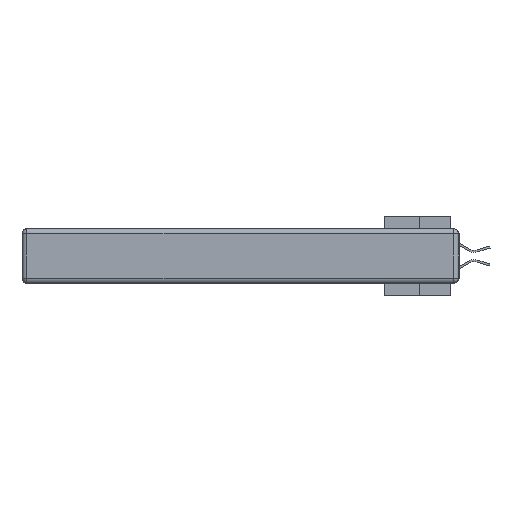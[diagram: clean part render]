
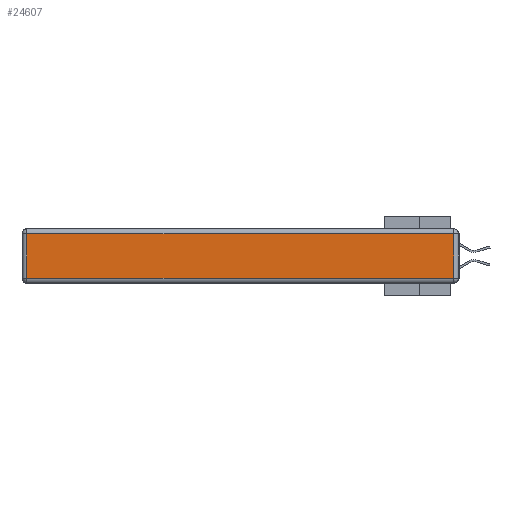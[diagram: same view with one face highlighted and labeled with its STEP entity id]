
A CAD part, left-side view. The second image highlights one B-rep face of the part: STEP entity #24607.
In plain terms, the highlighted planar face has unit normal (-1, 0, 0).
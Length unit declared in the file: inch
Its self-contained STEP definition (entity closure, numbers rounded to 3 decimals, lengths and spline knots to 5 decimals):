
#2348 = ORIENTED_EDGE ( 'NONE', *, *, #29073, .T. ) ;
#2840 = CARTESIAN_POINT ( 'NONE',  ( 0., 2.72, -0.343 ) ) ;
#3123 = CARTESIAN_POINT ( 'NONE',  ( 0., 2.72, -0.313 ) ) ;
#3370 = CARTESIAN_POINT ( 'NONE',  ( 0., 0., -0.343 ) ) ;
#4857 = LINE ( 'NONE', #33003, #16143 ) ;
#6246 = CARTESIAN_POINT ( 'NONE',  ( 0., 2.72, -0.03 ) ) ;
#7114 = VERTEX_POINT ( 'NONE', #3123 ) ;
#9445 = DIRECTION ( 'NONE',  ( 0., 1., 0. ) ) ;
#12820 = VECTOR ( 'NONE', #31341, 39.37008 ) ;
#13933 = EDGE_CURVE ( 'NONE', #24529, #7114, #23409, .T. ) ;
#14555 = EDGE_CURVE ( 'NONE', #23096, #25007, #15583, .T. ) ;
#15583 = LINE ( 'NONE', #30411, #22981 ) ;
#16143 = VECTOR ( 'NONE', #22887, 39.37008 ) ;
#16376 = ORIENTED_EDGE ( 'NONE', *, *, #13933, .T. ) ;
#17483 = CARTESIAN_POINT ( 'NONE',  ( 0., 0.03, -0.313 ) ) ;
#19044 = EDGE_CURVE ( 'NONE', #25007, #24529, #22059, .T. ) ;
#20258 = EDGE_LOOP ( 'NONE', ( #2348, #28731, #32077, #16376 ) ) ;
#20476 = CARTESIAN_POINT ( 'NONE',  ( 0., 2.75, -0.03 ) ) ;
#21233 = FACE_OUTER_BOUND ( 'NONE', #20258, .T. ) ;
#21402 = DIRECTION ( 'NONE',  ( -1., 0., 0. ) ) ;
#22059 = LINE ( 'NONE', #20476, #31390 ) ;
#22887 = DIRECTION ( 'NONE',  ( 0., -1., 0. ) ) ;
#22981 = VECTOR ( 'NONE', #25879, 39.37008 ) ;
#23096 = VERTEX_POINT ( 'NONE', #17483 ) ;
#23409 = LINE ( 'NONE', #2840, #12820 ) ;
#24529 = VERTEX_POINT ( 'NONE', #6246 ) ;
#24607 = ADVANCED_FACE ( 'NONE', ( #21233 ), #26481, .T. ) ;
#24687 = CARTESIAN_POINT ( 'NONE',  ( 0., 0.03, -0.03 ) ) ;
#25007 = VERTEX_POINT ( 'NONE', #24687 ) ;
#25879 = DIRECTION ( 'NONE',  ( 0., 0., 1. ) ) ;
#26481 = PLANE ( 'NONE',  #31069 ) ;
#28731 = ORIENTED_EDGE ( 'NONE', *, *, #14555, .T. ) ;
#29073 = EDGE_CURVE ( 'NONE', #7114, #23096, #4857, .T. ) ;
#29979 = DIRECTION ( 'NONE',  ( 0., 0., 1. ) ) ;
#30411 = CARTESIAN_POINT ( 'NONE',  ( 0., 0.03, -0.343 ) ) ;
#31069 = AXIS2_PLACEMENT_3D ( 'NONE', #3370, #21402, #29979 ) ;
#31341 = DIRECTION ( 'NONE',  ( 0., 0., -1. ) ) ;
#31390 = VECTOR ( 'NONE', #9445, 39.37008 ) ;
#32077 = ORIENTED_EDGE ( 'NONE', *, *, #19044, .T. ) ;
#33003 = CARTESIAN_POINT ( 'NONE',  ( 0., 0., -0.313 ) ) ;
